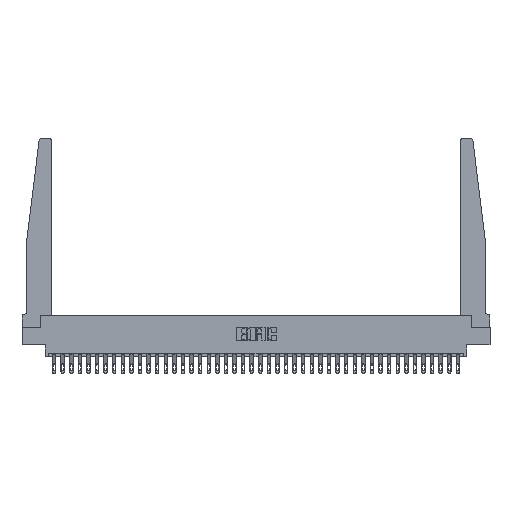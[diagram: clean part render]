
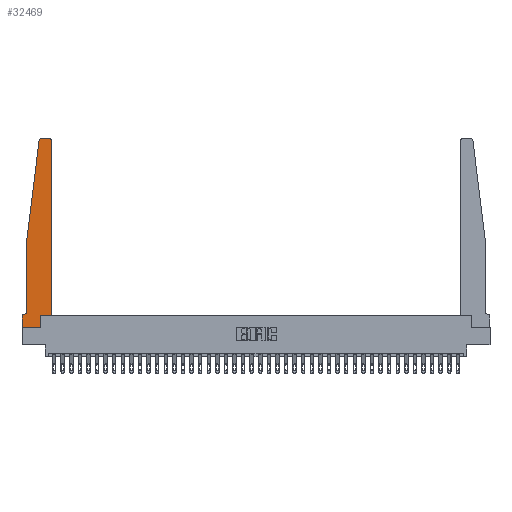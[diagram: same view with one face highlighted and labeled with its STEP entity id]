
A CAD part, top view. The second image highlights one B-rep face of the part: STEP entity #32469.
In plain terms, the highlighted planar face has unit normal (0, 0, 1).
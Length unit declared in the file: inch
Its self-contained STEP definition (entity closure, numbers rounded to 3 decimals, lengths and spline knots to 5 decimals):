
#164 = CARTESIAN_POINT ( 'NONE',  ( 0.425, 0.18, 0.37 ) ) ;
#1464 = CARTESIAN_POINT ( 'NONE',  ( 0., 0.1875, 0.37 ) ) ;
#1923 = DIRECTION ( 'NONE',  ( 1., 0., 0. ) ) ;
#1945 = VERTEX_POINT ( 'NONE', #31729 ) ;
#2460 = CARTESIAN_POINT ( 'NONE',  ( 0.065, 1.25, 0.37 ) ) ;
#2698 = CARTESIAN_POINT ( 'NONE',  ( 0., 0., 0.37 ) ) ;
#2803 = CARTESIAN_POINT ( 'NONE',  ( 0.24675, 2.72367, 0.37 ) ) ;
#2862 = ORIENTED_EDGE ( 'NONE', *, *, #23082, .T. ) ;
#3138 = DIRECTION ( 'NONE',  ( -0.122, -0.992, 0. ) ) ;
#3197 = CARTESIAN_POINT ( 'NONE',  ( 0.015, 0.2375, 0.37 ) ) ;
#3234 = CIRCLE ( 'NONE', #14418, 0.03 ) ;
#3303 = VECTOR ( 'NONE', #24293, 39.37008 ) ;
#3394 = VECTOR ( 'NONE', #3138, 39.37008 ) ;
#3516 = EDGE_CURVE ( 'NONE', #5055, #4382, #5293, .T. ) ;
#4187 = LINE ( 'NONE', #7698, #3303 ) ;
#4382 = VERTEX_POINT ( 'NONE', #9232 ) ;
#4651 = CARTESIAN_POINT ( 'NONE',  ( 0.2605, 0., 0.37 ) ) ;
#5055 = VERTEX_POINT ( 'NONE', #12475 ) ;
#5293 = LINE ( 'NONE', #164, #19182 ) ;
#5618 = VERTEX_POINT ( 'NONE', #1464 ) ;
#6003 = LINE ( 'NONE', #31635, #19878 ) ;
#6016 = DIRECTION ( 'NONE',  ( -1., 0., 0. ) ) ;
#6993 = CARTESIAN_POINT ( 'NONE',  ( 0.425, 0.18, 0.37 ) ) ;
#7413 = CARTESIAN_POINT ( 'NONE',  ( 0.25, 2.75, 0.37 ) ) ;
#7698 = CARTESIAN_POINT ( 'NONE',  ( 0.2605, 0.18, 0.37 ) ) ;
#7752 = EDGE_CURVE ( 'NONE', #23198, #10522, #21243, .T. ) ;
#8072 = ORIENTED_EDGE ( 'NONE', *, *, #8633, .T. ) ;
#8086 = LINE ( 'NONE', #7413, #28368 ) ;
#8551 = CARTESIAN_POINT ( 'NONE',  ( 0.27653, 2.72, 0.37 ) ) ;
#8633 = EDGE_CURVE ( 'NONE', #15825, #5618, #16850, .T. ) ;
#8678 = EDGE_CURVE ( 'NONE', #21413, #18207, #6003, .T. ) ;
#9232 = CARTESIAN_POINT ( 'NONE',  ( 0.425, 2.72, 0.37 ) ) ;
#9674 = ORIENTED_EDGE ( 'NONE', *, *, #29577, .T. ) ;
#9708 = DIRECTION ( 'NONE',  ( 0., -1., 0. ) ) ;
#9807 = DIRECTION ( 'NONE',  ( 1., 0., 0. ) ) ;
#10115 = CIRCLE ( 'NONE', #31275, 0.05 ) ;
#10522 = VERTEX_POINT ( 'NONE', #2803 ) ;
#10877 = CARTESIAN_POINT ( 'NONE',  ( 0., 0., 0.37 ) ) ;
#11343 = DIRECTION ( 'NONE',  ( 1., 0., 0. ) ) ;
#11379 = ORIENTED_EDGE ( 'NONE', *, *, #12854, .T. ) ;
#11474 = DIRECTION ( 'NONE',  ( 0., 1., 0. ) ) ;
#12475 = CARTESIAN_POINT ( 'NONE',  ( 0.425, 0.18, 0.37 ) ) ;
#12742 = VERTEX_POINT ( 'NONE', #4651 ) ;
#12854 = EDGE_CURVE ( 'NONE', #5618, #21473, #32032, .T. ) ;
#12930 = CARTESIAN_POINT ( 'NONE',  ( 0.2605, 0.18, 0.37 ) ) ;
#13388 = ORIENTED_EDGE ( 'NONE', *, *, #28583, .T. ) ;
#14243 = DIRECTION ( 'NONE',  ( 1., 0., 0. ) ) ;
#14267 = LINE ( 'NONE', #6993, #35329 ) ;
#14418 = AXIS2_PLACEMENT_3D ( 'NONE', #31053, #14555, #33776 ) ;
#14555 = DIRECTION ( 'NONE',  ( 0., 0., 1. ) ) ;
#15257 = EDGE_CURVE ( 'NONE', #21473, #12742, #18583, .T. ) ;
#15706 = CARTESIAN_POINT ( 'NONE',  ( 0.27653, 2.75, 0.37 ) ) ;
#15825 = VERTEX_POINT ( 'NONE', #35720 ) ;
#15973 = AXIS2_PLACEMENT_3D ( 'NONE', #8551, #27854, #11343 ) ;
#16850 = LINE ( 'NONE', #28874, #35347 ) ;
#16909 = EDGE_LOOP ( 'NONE', ( #22332, #21087, #33426, #32250, #28463, #8072, #11379, #30853, #13388, #2862, #25086, #9674 ) ) ;
#18207 = VERTEX_POINT ( 'NONE', #30006 ) ;
#18560 = DIRECTION ( 'NONE',  ( 0., 0., 1. ) ) ;
#18583 = LINE ( 'NONE', #22432, #25920 ) ;
#19083 = DIRECTION ( 'NONE',  ( 0., -1., 0. ) ) ;
#19182 = VECTOR ( 'NONE', #11474, 39.37008 ) ;
#19641 = EDGE_CURVE ( 'NONE', #18207, #15825, #10115, .T. ) ;
#19878 = VECTOR ( 'NONE', #9708, 39.37008 ) ;
#20004 = AXIS2_PLACEMENT_3D ( 'NONE', #35020, #18560, #1923 ) ;
#21087 = ORIENTED_EDGE ( 'NONE', *, *, #7752, .T. ) ;
#21243 = CIRCLE ( 'NONE', #15973, 0.03 ) ;
#21413 = VERTEX_POINT ( 'NONE', #2460 ) ;
#21473 = VERTEX_POINT ( 'NONE', #2698 ) ;
#22332 = ORIENTED_EDGE ( 'NONE', *, *, #29206, .T. ) ;
#22432 = CARTESIAN_POINT ( 'NONE',  ( 0., 0., 0.37 ) ) ;
#22610 = DIRECTION ( 'NONE',  ( 0., 0., -1. ) ) ;
#23082 = EDGE_CURVE ( 'NONE', #29925, #5055, #14267, .T. ) ;
#23198 = VERTEX_POINT ( 'NONE', #15706 ) ;
#24293 = DIRECTION ( 'NONE',  ( 0., 1., 0. ) ) ;
#24673 = LINE ( 'NONE', #33447, #3394 ) ;
#25086 = ORIENTED_EDGE ( 'NONE', *, *, #3516, .T. ) ;
#25920 = VECTOR ( 'NONE', #14243, 39.37008 ) ;
#26546 = EDGE_CURVE ( 'NONE', #10522, #21413, #24673, .T. ) ;
#27854 = DIRECTION ( 'NONE',  ( 0., 0., 1. ) ) ;
#28368 = VECTOR ( 'NONE', #29502, 39.37008 ) ;
#28463 = ORIENTED_EDGE ( 'NONE', *, *, #19641, .T. ) ;
#28583 = EDGE_CURVE ( 'NONE', #12742, #29925, #4187, .T. ) ;
#28874 = CARTESIAN_POINT ( 'NONE',  ( 0.065, 0.1875, 0.37 ) ) ;
#29206 = EDGE_CURVE ( 'NONE', #1945, #23198, #8086, .T. ) ;
#29502 = DIRECTION ( 'NONE',  ( -1., 0., 0. ) ) ;
#29507 = PLANE ( 'NONE',  #20004 ) ;
#29577 = EDGE_CURVE ( 'NONE', #4382, #1945, #3234, .T. ) ;
#29832 = FACE_OUTER_BOUND ( 'NONE', #16909, .T. ) ;
#29925 = VERTEX_POINT ( 'NONE', #12930 ) ;
#30006 = CARTESIAN_POINT ( 'NONE',  ( 0.065, 0.2375, 0.37 ) ) ;
#30853 = ORIENTED_EDGE ( 'NONE', *, *, #15257, .T. ) ;
#31053 = CARTESIAN_POINT ( 'NONE',  ( 0.395, 2.72, 0.37 ) ) ;
#31182 = VECTOR ( 'NONE', #19083, 39.37008 ) ;
#31275 = AXIS2_PLACEMENT_3D ( 'NONE', #3197, #22610, #6016 ) ;
#31635 = CARTESIAN_POINT ( 'NONE',  ( 0.065, 1.25, 0.37 ) ) ;
#31729 = CARTESIAN_POINT ( 'NONE',  ( 0.395, 2.75, 0.37 ) ) ;
#32032 = LINE ( 'NONE', #10877, #31182 ) ;
#32250 = ORIENTED_EDGE ( 'NONE', *, *, #8678, .T. ) ;
#32469 = ADVANCED_FACE ( 'NONE', ( #29832 ), #29507, .T. ) ;
#33426 = ORIENTED_EDGE ( 'NONE', *, *, #26546, .T. ) ;
#33447 = CARTESIAN_POINT ( 'NONE',  ( 0.065, 1.25, 0.37 ) ) ;
#33776 = DIRECTION ( 'NONE',  ( 1., 0., 0. ) ) ;
#34380 = DIRECTION ( 'NONE',  ( -1., 0., 0. ) ) ;
#35020 = CARTESIAN_POINT ( 'NONE',  ( 0., 0.1875, 0.37 ) ) ;
#35329 = VECTOR ( 'NONE', #9807, 39.37008 ) ;
#35347 = VECTOR ( 'NONE', #34380, 39.37008 ) ;
#35720 = CARTESIAN_POINT ( 'NONE',  ( 0.015, 0.1875, 0.37 ) ) ;
